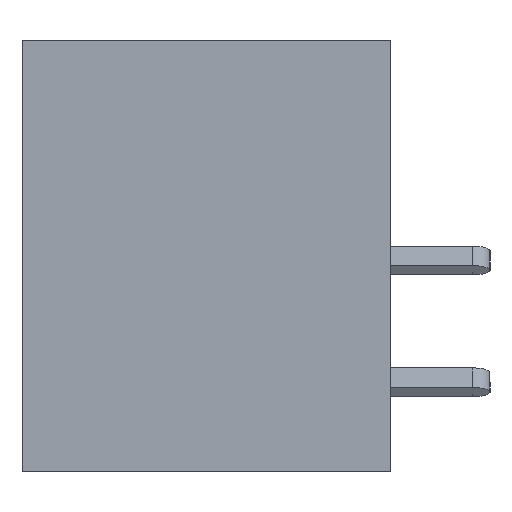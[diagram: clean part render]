
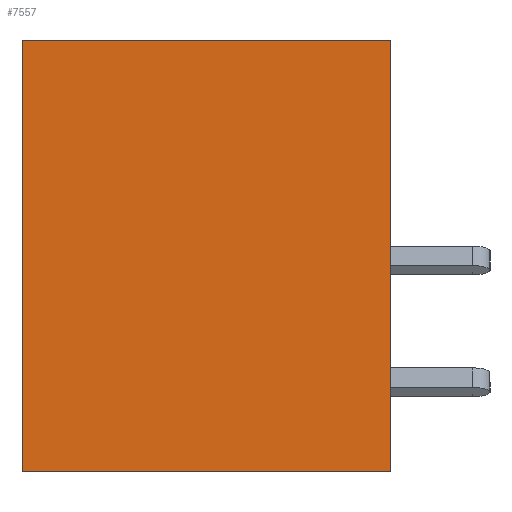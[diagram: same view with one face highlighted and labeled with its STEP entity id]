
A CAD part, left-side view. The second image highlights one B-rep face of the part: STEP entity #7557.
In plain terms, the highlighted planar face has unit normal (-1, 0, 0).
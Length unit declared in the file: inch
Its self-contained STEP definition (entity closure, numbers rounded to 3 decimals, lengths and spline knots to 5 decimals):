
#16 = VERTEX_POINT ( 'NONE', #11582 ) ;
#644 = LINE ( 'NONE', #5567, #16322 ) ;
#2106 = FACE_OUTER_BOUND ( 'NONE', #11055, .T. ) ;
#2283 = CARTESIAN_POINT ( 'NONE',  ( 0., 0.453, -0.531 ) ) ;
#2328 = LINE ( 'NONE', #14775, #12749 ) ;
#2986 = CARTESIAN_POINT ( 'NONE',  ( 0., 0.453, 0. ) ) ;
#3343 = AXIS2_PLACEMENT_3D ( 'NONE', #8817, #18406, #18272 ) ;
#3651 = VERTEX_POINT ( 'NONE', #6637 ) ;
#4223 = VECTOR ( 'NONE', #17987, 39.37008 ) ;
#4504 = EDGE_CURVE ( 'NONE', #13985, #3651, #6967, .T. ) ;
#5234 = CARTESIAN_POINT ( 'NONE',  ( 0., 0.453, 0. ) ) ;
#5567 = CARTESIAN_POINT ( 'NONE',  ( 0., 0.453, 0. ) ) ;
#6637 = CARTESIAN_POINT ( 'NONE',  ( 0., 0., -0.531 ) ) ;
#6967 = LINE ( 'NONE', #13312, #4223 ) ;
#7404 = LINE ( 'NONE', #5234, #19812 ) ;
#7557 = ADVANCED_FACE ( 'NONE', ( #2106 ), #16740, .F. ) ;
#8115 = EDGE_CURVE ( 'NONE', #3651, #16, #2328, .T. ) ;
#8601 = DIRECTION ( 'NONE',  ( 0., 0., 1. ) ) ;
#8817 = CARTESIAN_POINT ( 'NONE',  ( 0., 0.453, 0. ) ) ;
#11055 = EDGE_LOOP ( 'NONE', ( #14061, #13461, #20455, #12870 ) ) ;
#11185 = VERTEX_POINT ( 'NONE', #2986 ) ;
#11582 = CARTESIAN_POINT ( 'NONE',  ( 0., 0., 0. ) ) ;
#12749 = VECTOR ( 'NONE', #18042, 39.37008 ) ;
#12870 = ORIENTED_EDGE ( 'NONE', *, *, #4504, .T. ) ;
#13312 = CARTESIAN_POINT ( 'NONE',  ( 0., 0.453, -0.531 ) ) ;
#13461 = ORIENTED_EDGE ( 'NONE', *, *, #17747, .F. ) ;
#13664 = DIRECTION ( 'NONE',  ( 0., -1., 0. ) ) ;
#13985 = VERTEX_POINT ( 'NONE', #2283 ) ;
#14061 = ORIENTED_EDGE ( 'NONE', *, *, #8115, .T. ) ;
#14775 = CARTESIAN_POINT ( 'NONE',  ( 0., 0., 0. ) ) ;
#16322 = VECTOR ( 'NONE', #13664, 39.37008 ) ;
#16740 = PLANE ( 'NONE',  #3343 ) ;
#17622 = EDGE_CURVE ( 'NONE', #13985, #11185, #7404, .T. ) ;
#17747 = EDGE_CURVE ( 'NONE', #11185, #16, #644, .T. ) ;
#17987 = DIRECTION ( 'NONE',  ( 0., -1., 0. ) ) ;
#18042 = DIRECTION ( 'NONE',  ( 0., 0., 1. ) ) ;
#18272 = DIRECTION ( 'NONE',  ( 0., 0., -1. ) ) ;
#18406 = DIRECTION ( 'NONE',  ( 1., 0., 0. ) ) ;
#19812 = VECTOR ( 'NONE', #8601, 39.37008 ) ;
#20455 = ORIENTED_EDGE ( 'NONE', *, *, #17622, .F. ) ;
